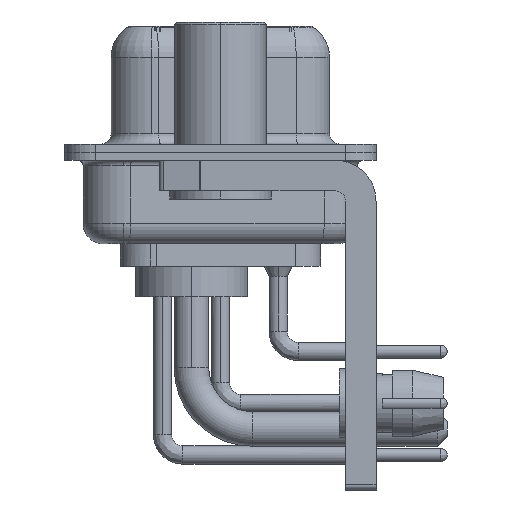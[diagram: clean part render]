
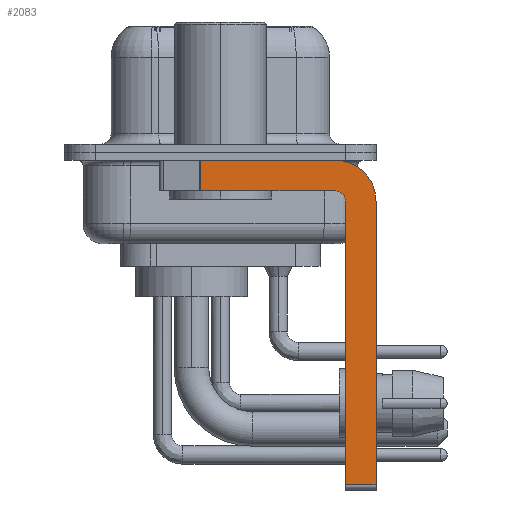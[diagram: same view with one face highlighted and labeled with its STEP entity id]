
A CAD part, left-side view. The second image highlights one B-rep face of the part: STEP entity #2083.
In plain terms, the highlighted planar face has unit normal (-1, 0, 0).
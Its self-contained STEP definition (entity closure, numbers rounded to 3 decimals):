
#51 = VECTOR ( 'NONE', #33685, 1000. ) ;
#1014 = CARTESIAN_POINT ( 'NONE',  ( -2.9, -5.65, -16.35 ) ) ;
#1217 = VECTOR ( 'NONE', #30800, 1000. ) ;
#2083 = ADVANCED_FACE ( 'NONE', ( #7549 ), #25840, .F. ) ;
#2653 = EDGE_LOOP ( 'NONE', ( #21152, #14424, #24065, #12634, #12899, #8299, #6697, #16140 ) ) ;
#2826 = CARTESIAN_POINT ( 'NONE',  ( -2.9, -5.65, -0.4 ) ) ;
#3921 = CARTESIAN_POINT ( 'NONE',  ( -2.9, -5.65, -2.4 ) ) ;
#4099 = DIRECTION ( 'NONE',  ( 0., 0., 1. ) ) ;
#5425 = DIRECTION ( 'NONE',  ( 0., 0., -1. ) ) ;
#5648 = CARTESIAN_POINT ( 'NONE',  ( -2.9, 0.978, -1.9 ) ) ;
#6540 = DIRECTION ( 'NONE',  ( 1., 0., 0. ) ) ;
#6697 = ORIENTED_EDGE ( 'NONE', *, *, #13899, .F. ) ;
#7549 = FACE_OUTER_BOUND ( 'NONE', #2653, .T. ) ;
#8299 = ORIENTED_EDGE ( 'NONE', *, *, #15492, .T. ) ;
#9897 = DIRECTION ( 'NONE',  ( 0., -1., 0. ) ) ;
#9959 = EDGE_CURVE ( 'NONE', #35062, #28671, #21444, .T. ) ;
#10463 = LINE ( 'NONE', #1014, #33216 ) ;
#11202 = DIRECTION ( 'NONE',  ( 1., 0., 0. ) ) ;
#11512 = VECTOR ( 'NONE', #30824, 1000. ) ;
#11549 = CARTESIAN_POINT ( 'NONE',  ( -2.9, -6.15, -16.35 ) ) ;
#12576 = LINE ( 'NONE', #13302, #11512 ) ;
#12634 = ORIENTED_EDGE ( 'NONE', *, *, #31246, .F. ) ;
#12899 = ORIENTED_EDGE ( 'NONE', *, *, #9959, .F. ) ;
#13165 = DIRECTION ( 'NONE',  ( -1., 0., 0. ) ) ;
#13294 = VERTEX_POINT ( 'NONE', #2826 ) ;
#13302 = CARTESIAN_POINT ( 'NONE',  ( -2.9, -7.65, -2.4 ) ) ;
#13899 = EDGE_CURVE ( 'NONE', #20708, #16854, #12576, .T. ) ;
#14424 = ORIENTED_EDGE ( 'NONE', *, *, #25933, .T. ) ;
#15492 = EDGE_CURVE ( 'NONE', #35062, #16854, #10463, .T. ) ;
#15630 = CARTESIAN_POINT ( 'NONE',  ( -2.9, 0.978, -0.4 ) ) ;
#15845 = CARTESIAN_POINT ( 'NONE',  ( -2.9, -6.15, -16.6 ) ) ;
#16140 = ORIENTED_EDGE ( 'NONE', *, *, #25311, .F. ) ;
#16854 = VERTEX_POINT ( 'NONE', #31553 ) ;
#17077 = VERTEX_POINT ( 'NONE', #27438 ) ;
#17161 = AXIS2_PLACEMENT_3D ( 'NONE', #31045, #11202, #5425 ) ;
#19052 = LINE ( 'NONE', #36969, #1217 ) ;
#19444 = LINE ( 'NONE', #33500, #51 ) ;
#19779 = CARTESIAN_POINT ( 'NONE',  ( -2.9, -7.65, -2.4 ) ) ;
#20227 = AXIS2_PLACEMENT_3D ( 'NONE', #3921, #13165, #33958 ) ;
#20708 = VERTEX_POINT ( 'NONE', #19779 ) ;
#21088 = AXIS2_PLACEMENT_3D ( 'NONE', #35446, #6540, #21180 ) ;
#21152 = ORIENTED_EDGE ( 'NONE', *, *, #33399, .F. ) ;
#21180 = DIRECTION ( 'NONE',  ( 0., 0., -1. ) ) ;
#21444 = LINE ( 'NONE', #15845, #35363 ) ;
#22384 = VECTOR ( 'NONE', #23565, 1000. ) ;
#23565 = DIRECTION ( 'NONE',  ( 0., 0., -1. ) ) ;
#24065 = ORIENTED_EDGE ( 'NONE', *, *, #32650, .F. ) ;
#24842 = VERTEX_POINT ( 'NONE', #15630 ) ;
#25218 = CARTESIAN_POINT ( 'NONE',  ( -2.9, -5.65, -1.9 ) ) ;
#25311 = EDGE_CURVE ( 'NONE', #13294, #20708, #29708, .T. ) ;
#25840 = PLANE ( 'NONE',  #17161 ) ;
#25933 = EDGE_CURVE ( 'NONE', #24842, #17077, #29352, .T. ) ;
#26769 = VERTEX_POINT ( 'NONE', #25218 ) ;
#27438 = CARTESIAN_POINT ( 'NONE',  ( -2.9, 0.978, -1.9 ) ) ;
#28671 = VERTEX_POINT ( 'NONE', #29846 ) ;
#29352 = LINE ( 'NONE', #5648, #22384 ) ;
#29708 = CIRCLE ( 'NONE', #21088, 2. ) ;
#29846 = CARTESIAN_POINT ( 'NONE',  ( -2.9, -6.15, -2.4 ) ) ;
#30800 = DIRECTION ( 'NONE',  ( 0., 1., 0. ) ) ;
#30824 = DIRECTION ( 'NONE',  ( 0., 0., -1. ) ) ;
#31045 = CARTESIAN_POINT ( 'NONE',  ( -2.9, -5.65, -2.4 ) ) ;
#31246 = EDGE_CURVE ( 'NONE', #28671, #26769, #34990, .T. ) ;
#31553 = CARTESIAN_POINT ( 'NONE',  ( -2.9, -7.65, -16.35 ) ) ;
#32650 = EDGE_CURVE ( 'NONE', #26769, #17077, #19052, .T. ) ;
#33216 = VECTOR ( 'NONE', #9897, 1000. ) ;
#33399 = EDGE_CURVE ( 'NONE', #24842, #13294, #19444, .T. ) ;
#33500 = CARTESIAN_POINT ( 'NONE',  ( -2.9, 3., -0.4 ) ) ;
#33685 = DIRECTION ( 'NONE',  ( 0., -1., 0. ) ) ;
#33958 = DIRECTION ( 'NONE',  ( 0., 0., 1. ) ) ;
#34990 = CIRCLE ( 'NONE', #20227, 0.5 ) ;
#35062 = VERTEX_POINT ( 'NONE', #11549 ) ;
#35363 = VECTOR ( 'NONE', #4099, 1000. ) ;
#35446 = CARTESIAN_POINT ( 'NONE',  ( -2.9, -5.65, -2.4 ) ) ;
#36969 = CARTESIAN_POINT ( 'NONE',  ( -2.9, -5.65, -1.9 ) ) ;
